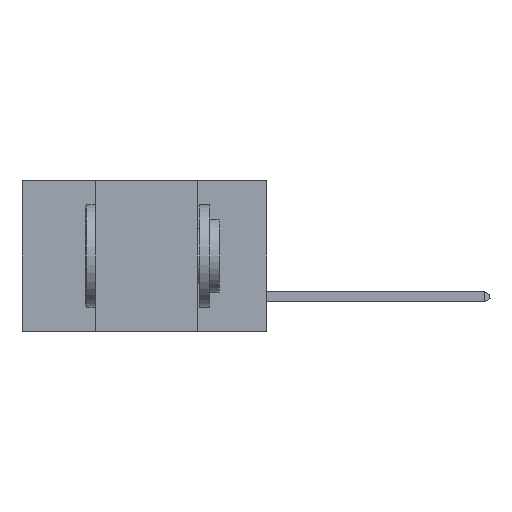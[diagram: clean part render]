
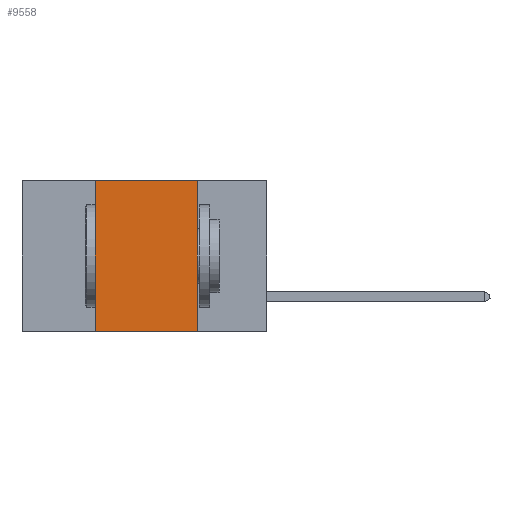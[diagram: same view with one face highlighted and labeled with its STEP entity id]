
A CAD part, left-side view. The second image highlights one B-rep face of the part: STEP entity #9558.
In plain terms, the highlighted planar face has unit normal (-1, 0, 0).
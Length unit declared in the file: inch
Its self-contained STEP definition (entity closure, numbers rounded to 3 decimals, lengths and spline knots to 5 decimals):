
#421 = ORIENTED_EDGE ( 'NONE', *, *, #681, .F. ) ;
#585 = VERTEX_POINT ( 'NONE', #10839 ) ;
#679 = DIRECTION ( 'NONE',  ( 0., 0., 1. ) ) ;
#681 = EDGE_CURVE ( 'NONE', #5754, #6167, #10211, .T. ) ;
#922 = DIRECTION ( 'NONE',  ( 0., 0., -1. ) ) ;
#1140 = FACE_OUTER_BOUND ( 'NONE', #8336, .T. ) ;
#1337 = VECTOR ( 'NONE', #679, 39.37008 ) ;
#1387 = DIRECTION ( 'NONE',  ( 0., -1., 0. ) ) ;
#2190 = VECTOR ( 'NONE', #13518, 39.37008 ) ;
#4300 = ORIENTED_EDGE ( 'NONE', *, *, #9699, .F. ) ;
#4423 = EDGE_CURVE ( 'NONE', #5754, #8143, #4609, .T. ) ;
#4609 = LINE ( 'NONE', #7696, #7398 ) ;
#4638 = VECTOR ( 'NONE', #1387, 39.37008 ) ;
#5223 = CARTESIAN_POINT ( 'NONE',  ( 0., 0.6, 0. ) ) ;
#5691 = CARTESIAN_POINT ( 'NONE',  ( 0., 0.6, 0. ) ) ;
#5754 = VERTEX_POINT ( 'NONE', #9985 ) ;
#6167 = VERTEX_POINT ( 'NONE', #6678 ) ;
#6678 = CARTESIAN_POINT ( 'NONE',  ( 0., 0.42, 0. ) ) ;
#6959 = CARTESIAN_POINT ( 'NONE',  ( 0., 0.17, 0. ) ) ;
#7398 = VECTOR ( 'NONE', #8745, 39.37008 ) ;
#7507 = DIRECTION ( 'NONE',  ( 1., 0., 0. ) ) ;
#7696 = CARTESIAN_POINT ( 'NONE',  ( 0., 0.6, -0.37 ) ) ;
#8072 = CARTESIAN_POINT ( 'NONE',  ( 0., 0.17, -0.37 ) ) ;
#8143 = VERTEX_POINT ( 'NONE', #8072 ) ;
#8336 = EDGE_LOOP ( 'NONE', ( #4300, #12684, #421, #11290 ) ) ;
#8606 = EDGE_CURVE ( 'NONE', #6167, #585, #13725, .T. ) ;
#8745 = DIRECTION ( 'NONE',  ( 0., -1., 0. ) ) ;
#9494 = AXIS2_PLACEMENT_3D ( 'NONE', #5223, #7507, #922 ) ;
#9558 = ADVANCED_FACE ( 'NONE', ( #1140 ), #9629, .F. ) ;
#9629 = PLANE ( 'NONE',  #9494 ) ;
#9699 = EDGE_CURVE ( 'NONE', #585, #8143, #11070, .T. ) ;
#9985 = CARTESIAN_POINT ( 'NONE',  ( 0., 0.42, -0.37 ) ) ;
#10211 = LINE ( 'NONE', #14147, #1337 ) ;
#10839 = CARTESIAN_POINT ( 'NONE',  ( 0., 0.17, 0. ) ) ;
#11070 = LINE ( 'NONE', #6959, #2190 ) ;
#11290 = ORIENTED_EDGE ( 'NONE', *, *, #4423, .T. ) ;
#12684 = ORIENTED_EDGE ( 'NONE', *, *, #8606, .F. ) ;
#13518 = DIRECTION ( 'NONE',  ( 0., 0., -1. ) ) ;
#13725 = LINE ( 'NONE', #5691, #4638 ) ;
#14147 = CARTESIAN_POINT ( 'NONE',  ( 0., 0.42, 0. ) ) ;
